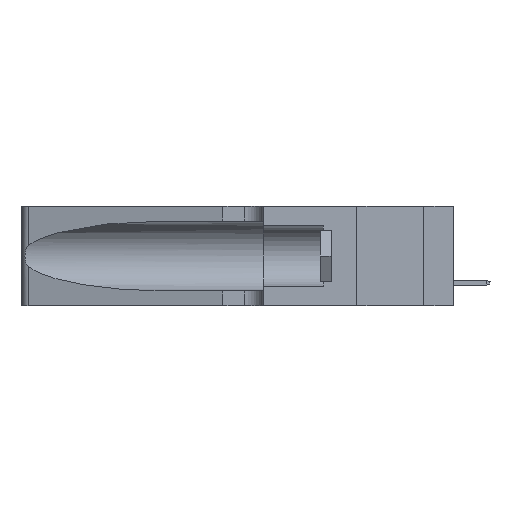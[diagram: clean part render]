
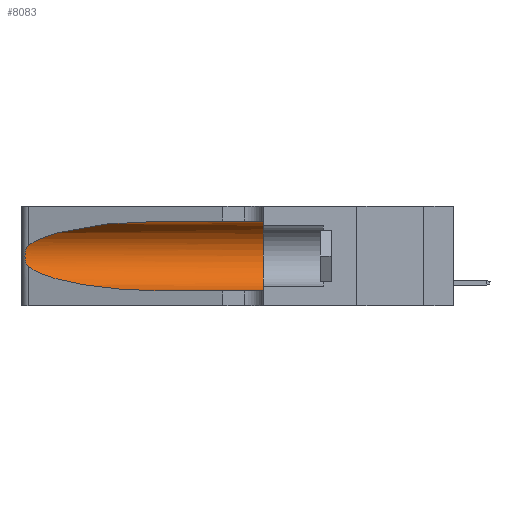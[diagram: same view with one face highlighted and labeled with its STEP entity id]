
A CAD part, left-side view. The second image highlights one B-rep face of the part: STEP entity #8083.
In plain terms, the highlighted cylindrical face has radius 3.308 mm (diameter 6.617 mm), a partial arc.
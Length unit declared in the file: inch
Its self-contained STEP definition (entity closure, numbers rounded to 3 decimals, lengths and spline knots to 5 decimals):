
#25 = CARTESIAN_POINT ( 'NONE',  ( 0.25639, 1.23186, 0.15144 ) ) ;
#428 = EDGE_CURVE ( 'NONE', #4204, #15460, #17805, .T. ) ;
#900 = DIRECTION ( 'NONE',  ( 0., -1., 0. ) ) ;
#2365 = ORIENTED_EDGE ( 'NONE', *, *, #428, .T. ) ;
#2370 = CARTESIAN_POINT ( 'NONE',  ( 0.1305, 0.35, 0.05475 ) ) ;
#2574 = CARTESIAN_POINT ( 'NONE',  ( 0.25787, 1.23484, 0.2124 ) ) ;
#2777 = CARTESIAN_POINT ( 'NONE',  ( 0.25487, 1.22718, 0.22369 ) ) ;
#3887 = DIRECTION ( 'NONE',  ( 0., 0., 1. ) ) ;
#4204 = VERTEX_POINT ( 'NONE', #11603 ) ;
#4283 = CARTESIAN_POINT ( 'NONE',  ( 0.25487, 1.22718, 0.14631 ) ) ;
#4831 = CARTESIAN_POINT ( 'NONE',  ( 0.1305, 1.61858, 0.05475 ) ) ;
#5686 = DIRECTION ( 'NONE',  ( 0., -1., 0. ) ) ;
#6278 = VERTEX_POINT ( 'NONE', #11152 ) ;
#7997 = ORIENTED_EDGE ( 'NONE', *, *, #8593, .T. ) ;
#8083 = ADVANCED_FACE ( 'NONE', ( #17261 ), #19453, .F. ) ;
#8197 = CARTESIAN_POINT ( 'NONE',  ( 0.26018, 1.23835, 0.19895 ) ) ;
#8268 = VERTEX_POINT ( 'NONE', #23407 ) ;
#8391 = CARTESIAN_POINT ( 'NONE',  ( 0.18966, 0.96281, 0.31525 ) ) ;
#8575 = EDGE_CURVE ( 'NONE', #4204, #18041, #18785, .T. ) ;
#8593 = EDGE_CURVE ( 'NONE', #8268, #21372, #29663, .T. ) ;
#9892 = CARTESIAN_POINT ( 'NONE',  ( 0.18966, 0.96281, 0.05475 ) ) ;
#10482 = B_SPLINE_CURVE_WITH_KNOTS ( 'NONE', 3,
 ( #10554, #21426, #32494, #2574, #16704, #8197, #27759, #21785, #30132, #21972, #24685, #25, #11087, #24862 ),
 .UNSPECIFIED., .F., .F.,
 ( 4, 2, 2, 2, 2, 2, 4 ),
 ( 0., 0.00027, 0.00053, 0.00107, 0.0016, 0.00187, 0.00214 ),
 .UNSPECIFIED. ) ;
#10554 = CARTESIAN_POINT ( 'NONE',  ( 0.25487, 1.22718, 0.22369 ) ) ;
#11087 = CARTESIAN_POINT ( 'NONE',  ( 0.25555, 1.22993, 0.14849 ) ) ;
#11152 = CARTESIAN_POINT ( 'NONE',  ( 0.25487, 1.22718, 0.14631 ) ) ;
#11603 = CARTESIAN_POINT ( 'NONE',  ( 0.1305, 0.72297, 0.31525 ) ) ;
#12620 = CARTESIAN_POINT ( 'NONE',  ( 0.1305, 0.72297, 0.05475 ) ) ;
#13733 = CIRCLE ( 'NONE', #29929, 0.13025 ) ;
#14106 =( BOUNDED_CURVE ( )  B_SPLINE_CURVE ( 3, ( #4283, #31668, #9892, #12620 ),
 .UNSPECIFIED., .F., .F. ) 
 B_SPLINE_CURVE_WITH_KNOTS ( ( 4, 4 ),
 ( 3.44316, 4.71239 ),
 .UNSPECIFIED. ) 
 CURVE ( )  GEOMETRIC_REPRESENTATION_ITEM ( )  RATIONAL_B_SPLINE_CURVE ( ( 1., 0.87, 0.87, 1. ) ) 
 REPRESENTATION_ITEM ( '' )  );
#14191 = DIRECTION ( 'NONE',  ( 0., 0., -1. ) ) ;
#15460 = VERTEX_POINT ( 'NONE', #16969 ) ;
#16704 = CARTESIAN_POINT ( 'NONE',  ( 0.25854, 1.2359, 0.20912 ) ) ;
#16969 = CARTESIAN_POINT ( 'NONE',  ( 0.25487, 1.22718, 0.22369 ) ) ;
#17261 = FACE_OUTER_BOUND ( 'NONE', #32326, .T. ) ;
#17805 =( BOUNDED_CURVE ( )  B_SPLINE_CURVE ( 3, ( #32883, #8391, #19280, #2777 ),
 .UNSPECIFIED., .F., .T. ) 
 B_SPLINE_CURVE_WITH_KNOTS ( ( 4, 4 ),
 ( 1.5708, 2.84003 ),
 .UNSPECIFIED. ) 
 CURVE ( )  GEOMETRIC_REPRESENTATION_ITEM ( )  RATIONAL_B_SPLINE_CURVE ( ( 1., 0.87, 0.87, 1. ) ) 
 REPRESENTATION_ITEM ( '' )  );
#18041 = VERTEX_POINT ( 'NONE', #27755 ) ;
#18785 = LINE ( 'NONE', #31545, #32552 ) ;
#19280 = CARTESIAN_POINT ( 'NONE',  ( 0.2373, 1.15595, 0.28018 ) ) ;
#19453 = CYLINDRICAL_SURFACE ( 'NONE', #26171, 0.13025 ) ;
#21372 = VERTEX_POINT ( 'NONE', #2370 ) ;
#21426 = CARTESIAN_POINT ( 'NONE',  ( 0.25555, 1.22994, 0.2215 ) ) ;
#21785 = CARTESIAN_POINT ( 'NONE',  ( 0.26075, 1.23896, 0.178 ) ) ;
#21972 = CARTESIAN_POINT ( 'NONE',  ( 0.25856, 1.23593, 0.16098 ) ) ;
#22516 = CARTESIAN_POINT ( 'NONE',  ( 0.1305, 1.61858, 0.185 ) ) ;
#22545 = ORIENTED_EDGE ( 'NONE', *, *, #28897, .T. ) ;
#23407 = CARTESIAN_POINT ( 'NONE',  ( 0.1305, 0.72297, 0.05475 ) ) ;
#24176 = EDGE_CURVE ( 'NONE', #18041, #21372, #13733, .T. ) ;
#24685 = CARTESIAN_POINT ( 'NONE',  ( 0.25789, 1.23486, 0.15765 ) ) ;
#24862 = CARTESIAN_POINT ( 'NONE',  ( 0.25487, 1.22718, 0.14631 ) ) ;
#25013 = EDGE_CURVE ( 'NONE', #6278, #8268, #14106, .T. ) ;
#25775 = ORIENTED_EDGE ( 'NONE', *, *, #25013, .T. ) ;
#26171 = AXIS2_PLACEMENT_3D ( 'NONE', #22516, #5686, #14191 ) ;
#27755 = CARTESIAN_POINT ( 'NONE',  ( 0.1305, 0.35, 0.31525 ) ) ;
#27759 = CARTESIAN_POINT ( 'NONE',  ( 0.26075, 1.23896, 0.19203 ) ) ;
#28712 = DIRECTION ( 'NONE',  ( 0., 1., 0. ) ) ;
#28897 = EDGE_CURVE ( 'NONE', #15460, #6278, #10482, .T. ) ;
#29663 = LINE ( 'NONE', #4831, #34878 ) ;
#29929 = AXIS2_PLACEMENT_3D ( 'NONE', #34335, #28712, #3887 ) ;
#30132 = CARTESIAN_POINT ( 'NONE',  ( 0.26017, 1.23833, 0.17102 ) ) ;
#31545 = CARTESIAN_POINT ( 'NONE',  ( 0.1305, 1.61858, 0.31525 ) ) ;
#31668 = CARTESIAN_POINT ( 'NONE',  ( 0.2373, 1.15595, 0.08982 ) ) ;
#31722 = ORIENTED_EDGE ( 'NONE', *, *, #8575, .F. ) ;
#32214 = DIRECTION ( 'NONE',  ( 0., -1., 0. ) ) ;
#32326 = EDGE_LOOP ( 'NONE', ( #2365, #22545, #25775, #7997, #34539, #31722 ) ) ;
#32494 = CARTESIAN_POINT ( 'NONE',  ( 0.25639, 1.23184, 0.21858 ) ) ;
#32552 = VECTOR ( 'NONE', #32214, 39.37008 ) ;
#32883 = CARTESIAN_POINT ( 'NONE',  ( 0.1305, 0.72297, 0.31525 ) ) ;
#34335 = CARTESIAN_POINT ( 'NONE',  ( 0.1305, 0.35, 0.185 ) ) ;
#34539 = ORIENTED_EDGE ( 'NONE', *, *, #24176, .F. ) ;
#34878 = VECTOR ( 'NONE', #900, 39.37008 ) ;
